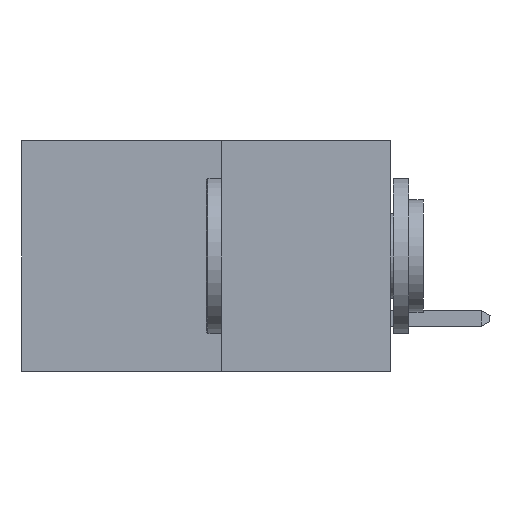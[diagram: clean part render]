
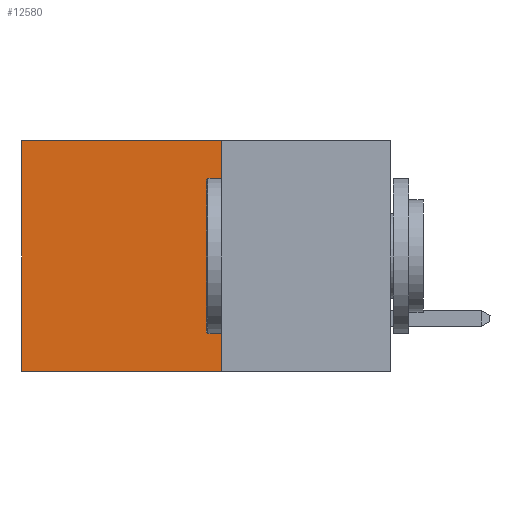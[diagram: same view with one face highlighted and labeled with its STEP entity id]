
A CAD part, left-side view. The second image highlights one B-rep face of the part: STEP entity #12580.
In plain terms, the highlighted planar face has unit normal (-1, 0, 0).
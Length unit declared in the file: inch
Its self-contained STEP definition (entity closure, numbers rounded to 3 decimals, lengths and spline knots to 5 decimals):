
#123 = DIRECTION ( 'NONE',  ( 0., 1., 0. ) ) ;
#127 = CARTESIAN_POINT ( 'NONE',  ( 0.277, 0.27, -0.37 ) ) ;
#442 = CARTESIAN_POINT ( 'NONE',  ( 0.277, 0.27, -0.37 ) ) ;
#1646 = ORIENTED_EDGE ( 'NONE', *, *, #8763, .T. ) ;
#3135 = DIRECTION ( 'NONE',  ( 0., 1., 0. ) ) ;
#3192 = CARTESIAN_POINT ( 'NONE',  ( 0.277, 0.27, 0. ) ) ;
#3799 = VECTOR ( 'NONE', #9237, 39.37008 ) ;
#6991 = CARTESIAN_POINT ( 'NONE',  ( 0.277, 0.27, -0.37 ) ) ;
#7818 = LINE ( 'NONE', #20929, #16785 ) ;
#8745 = VERTEX_POINT ( 'NONE', #9618 ) ;
#8763 = EDGE_CURVE ( 'NONE', #8745, #12872, #13936, .T. ) ;
#8810 = DIRECTION ( 'NONE',  ( 0., 0., -1. ) ) ;
#9237 = DIRECTION ( 'NONE',  ( 0., 0., -1. ) ) ;
#9357 = EDGE_CURVE ( 'NONE', #13798, #8745, #14189, .T. ) ;
#9608 = VERTEX_POINT ( 'NONE', #442 ) ;
#9617 = EDGE_CURVE ( 'NONE', #9608, #12872, #13337, .T. ) ;
#9618 = CARTESIAN_POINT ( 'NONE',  ( 0.277, 0.59, 0. ) ) ;
#9708 = VECTOR ( 'NONE', #123, 39.37008 ) ;
#10919 = EDGE_LOOP ( 'NONE', ( #1646, #21041, #19637, #18221 ) ) ;
#12429 = EDGE_CURVE ( 'NONE', #13798, #9608, #7818, .T. ) ;
#12580 = ADVANCED_FACE ( 'NONE', ( #13951 ), #17747, .F. ) ;
#12872 = VERTEX_POINT ( 'NONE', #23127 ) ;
#13337 = LINE ( 'NONE', #127, #9708 ) ;
#13564 = CARTESIAN_POINT ( 'NONE',  ( 0.277, 0.59, -0.37 ) ) ;
#13798 = VERTEX_POINT ( 'NONE', #22100 ) ;
#13936 = LINE ( 'NONE', #13564, #3799 ) ;
#13951 = FACE_OUTER_BOUND ( 'NONE', #10919, .T. ) ;
#14189 = LINE ( 'NONE', #3192, #18403 ) ;
#16785 = VECTOR ( 'NONE', #22711, 39.37008 ) ;
#17747 = PLANE ( 'NONE',  #18523 ) ;
#18221 = ORIENTED_EDGE ( 'NONE', *, *, #9357, .T. ) ;
#18403 = VECTOR ( 'NONE', #3135, 39.37008 ) ;
#18523 = AXIS2_PLACEMENT_3D ( 'NONE', #6991, #19504, #8810 ) ;
#19504 = DIRECTION ( 'NONE',  ( 1., 0., 0. ) ) ;
#19637 = ORIENTED_EDGE ( 'NONE', *, *, #12429, .F. ) ;
#20929 = CARTESIAN_POINT ( 'NONE',  ( 0.277, 0.27, -0.37 ) ) ;
#21041 = ORIENTED_EDGE ( 'NONE', *, *, #9617, .F. ) ;
#22100 = CARTESIAN_POINT ( 'NONE',  ( 0.277, 0.27, 0. ) ) ;
#22711 = DIRECTION ( 'NONE',  ( 0., 0., -1. ) ) ;
#23127 = CARTESIAN_POINT ( 'NONE',  ( 0.277, 0.59, -0.37 ) ) ;
